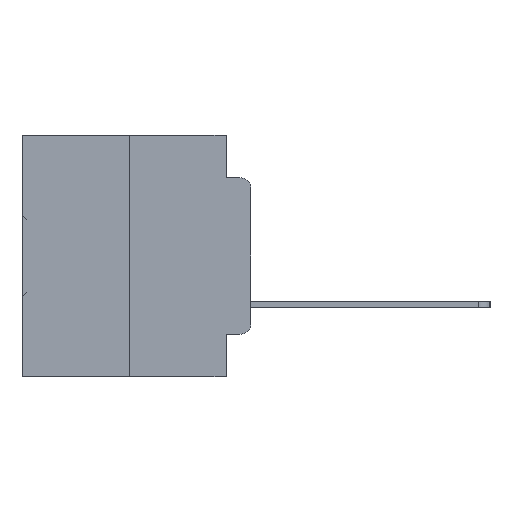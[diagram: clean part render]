
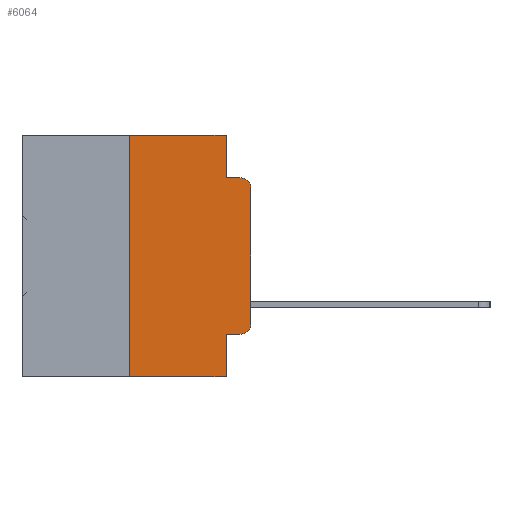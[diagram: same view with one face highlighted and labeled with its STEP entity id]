
A CAD part, left-side view. The second image highlights one B-rep face of the part: STEP entity #6064.
In plain terms, the highlighted planar face has unit normal (-1, 0, 0).
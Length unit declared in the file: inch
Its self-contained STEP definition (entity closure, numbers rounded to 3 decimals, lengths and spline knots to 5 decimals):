
#26 = EDGE_CURVE ( 'NONE', #13650, #2940, #5682, .T. ) ;
#1029 = CARTESIAN_POINT ( 'NONE',  ( 0., 0.473, 0. ) ) ;
#2264 = VERTEX_POINT ( 'NONE', #13331 ) ;
#2592 = DIRECTION ( 'NONE',  ( 0., -1., 0. ) ) ;
#2940 = VERTEX_POINT ( 'NONE', #18218 ) ;
#3049 = CARTESIAN_POINT ( 'NONE',  ( 0., 0.25, 0. ) ) ;
#3906 = DIRECTION ( 'NONE',  ( 0., 0., -1. ) ) ;
#4088 = VECTOR ( 'NONE', #32008, 39.37008 ) ;
#4770 = VECTOR ( 'NONE', #38302, 39.37008 ) ;
#4924 = LINE ( 'NONE', #1029, #24944 ) ;
#5491 = CARTESIAN_POINT ( 'NONE',  ( 0., 0.051, -0.0885 ) ) ;
#5682 = LINE ( 'NONE', #24593, #11751 ) ;
#5782 = CARTESIAN_POINT ( 'NONE',  ( 0., 0.473, -0.5 ) ) ;
#6064 = ADVANCED_FACE ( 'NONE', ( #22327 ), #7321, .F. ) ;
#6361 = ORIENTED_EDGE ( 'NONE', *, *, #26, .F. ) ;
#6759 = VERTEX_POINT ( 'NONE', #7401 ) ;
#6837 = ORIENTED_EDGE ( 'NONE', *, *, #21805, .F. ) ;
#7217 = LINE ( 'NONE', #35294, #13285 ) ;
#7321 = PLANE ( 'NONE',  #13993 ) ;
#7401 = CARTESIAN_POINT ( 'NONE',  ( 0., 0.051, -0.5 ) ) ;
#8244 = ORIENTED_EDGE ( 'NONE', *, *, #15145, .F. ) ;
#10187 = DIRECTION ( 'NONE',  ( -1., 0., 0. ) ) ;
#10211 = EDGE_CURVE ( 'NONE', #2940, #2264, #31686, .T. ) ;
#11398 = VECTOR ( 'NONE', #32497, 39.37008 ) ;
#11681 = ORIENTED_EDGE ( 'NONE', *, *, #28677, .T. ) ;
#11751 = VECTOR ( 'NONE', #12096, 39.37008 ) ;
#11891 = VERTEX_POINT ( 'NONE', #34327 ) ;
#12038 = LINE ( 'NONE', #20081, #4088 ) ;
#12096 = DIRECTION ( 'NONE',  ( 0., 0., -1. ) ) ;
#12976 = EDGE_CURVE ( 'NONE', #22625, #13650, #4924, .T. ) ;
#13013 = EDGE_CURVE ( 'NONE', #27899, #11891, #17045, .T. ) ;
#13285 = VECTOR ( 'NONE', #2592, 39.37008 ) ;
#13328 = DIRECTION ( 'NONE',  ( 0., 0., -1. ) ) ;
#13331 = CARTESIAN_POINT ( 'NONE',  ( 0., 0.02, -0.0885 ) ) ;
#13650 = VERTEX_POINT ( 'NONE', #36954 ) ;
#13752 = CARTESIAN_POINT ( 'NONE',  ( 0., 0.02, -0.1085 ) ) ;
#13993 = AXIS2_PLACEMENT_3D ( 'NONE', #28125, #31117, #13328 ) ;
#14263 = EDGE_CURVE ( 'NONE', #11891, #25321, #19337, .T. ) ;
#15145 = EDGE_CURVE ( 'NONE', #25417, #6759, #36969, .T. ) ;
#15212 = ORIENTED_EDGE ( 'NONE', *, *, #10211, .F. ) ;
#16430 = VERTEX_POINT ( 'NONE', #36908 ) ;
#16735 = DIRECTION ( 'NONE',  ( 0., 0., -1. ) ) ;
#16821 = ORIENTED_EDGE ( 'NONE', *, *, #23664, .T. ) ;
#17045 = CIRCLE ( 'NONE', #23667, 0.02 ) ;
#17542 = CARTESIAN_POINT ( 'NONE',  ( 0., 0., 0. ) ) ;
#18218 = CARTESIAN_POINT ( 'NONE',  ( 0., 0.051, -0.0885 ) ) ;
#18728 = EDGE_CURVE ( 'NONE', #25321, #2264, #36691, .T. ) ;
#18927 = DIRECTION ( 'NONE',  ( 0., -1., 0. ) ) ;
#19337 = LINE ( 'NONE', #17542, #11398 ) ;
#19529 = CARTESIAN_POINT ( 'NONE',  ( 0., 0.02, -0.4115 ) ) ;
#20081 = CARTESIAN_POINT ( 'NONE',  ( 0., 0.25, 0. ) ) ;
#21805 = EDGE_CURVE ( 'NONE', #16430, #22625, #12038, .T. ) ;
#22327 = FACE_OUTER_BOUND ( 'NONE', #28710, .T. ) ;
#22625 = VERTEX_POINT ( 'NONE', #3049 ) ;
#22799 = AXIS2_PLACEMENT_3D ( 'NONE', #13752, #34534, #16735 ) ;
#22805 = ORIENTED_EDGE ( 'NONE', *, *, #12976, .F. ) ;
#23629 = DIRECTION ( 'NONE',  ( 0., -1., 0. ) ) ;
#23664 = EDGE_CURVE ( 'NONE', #25417, #27899, #7217, .T. ) ;
#23667 = AXIS2_PLACEMENT_3D ( 'NONE', #28005, #10187, #31002 ) ;
#24418 = ORIENTED_EDGE ( 'NONE', *, *, #18728, .T. ) ;
#24593 = CARTESIAN_POINT ( 'NONE',  ( 0., 0.051, 0. ) ) ;
#24944 = VECTOR ( 'NONE', #18927, 39.37008 ) ;
#25321 = VERTEX_POINT ( 'NONE', #28383 ) ;
#25417 = VERTEX_POINT ( 'NONE', #29403 ) ;
#26112 = ORIENTED_EDGE ( 'NONE', *, *, #14263, .T. ) ;
#27747 = CARTESIAN_POINT ( 'NONE',  ( 0., 0.051, 0. ) ) ;
#27899 = VERTEX_POINT ( 'NONE', #19529 ) ;
#28005 = CARTESIAN_POINT ( 'NONE',  ( 0., 0.02, -0.3915 ) ) ;
#28125 = CARTESIAN_POINT ( 'NONE',  ( 0., 0.473, 0. ) ) ;
#28383 = CARTESIAN_POINT ( 'NONE',  ( 0., 0., -0.1085 ) ) ;
#28677 = EDGE_CURVE ( 'NONE', #16430, #6759, #28760, .T. ) ;
#28710 = EDGE_LOOP ( 'NONE', ( #26112, #24418, #15212, #6361, #22805, #6837, #11681, #8244, #16821, #30155 ) ) ;
#28760 = LINE ( 'NONE', #5782, #36718 ) ;
#29018 = VECTOR ( 'NONE', #3906, 39.37008 ) ;
#29403 = CARTESIAN_POINT ( 'NONE',  ( 0., 0.051, -0.4115 ) ) ;
#30155 = ORIENTED_EDGE ( 'NONE', *, *, #13013, .T. ) ;
#31002 = DIRECTION ( 'NONE',  ( 0., 0., -1. ) ) ;
#31117 = DIRECTION ( 'NONE',  ( 1., 0., 0. ) ) ;
#31686 = LINE ( 'NONE', #5491, #4770 ) ;
#32008 = DIRECTION ( 'NONE',  ( 0., 0., 1. ) ) ;
#32497 = DIRECTION ( 'NONE',  ( 0., 0., 1. ) ) ;
#34327 = CARTESIAN_POINT ( 'NONE',  ( 0., 0., -0.3915 ) ) ;
#34534 = DIRECTION ( 'NONE',  ( -1., 0., 0. ) ) ;
#35294 = CARTESIAN_POINT ( 'NONE',  ( 0., 0.051, -0.4115 ) ) ;
#36691 = CIRCLE ( 'NONE', #22799, 0.02 ) ;
#36718 = VECTOR ( 'NONE', #23629, 39.37008 ) ;
#36908 = CARTESIAN_POINT ( 'NONE',  ( 0., 0.25, -0.5 ) ) ;
#36954 = CARTESIAN_POINT ( 'NONE',  ( 0., 0.051, 0. ) ) ;
#36969 = LINE ( 'NONE', #27747, #29018 ) ;
#38302 = DIRECTION ( 'NONE',  ( 0., -1., 0. ) ) ;
